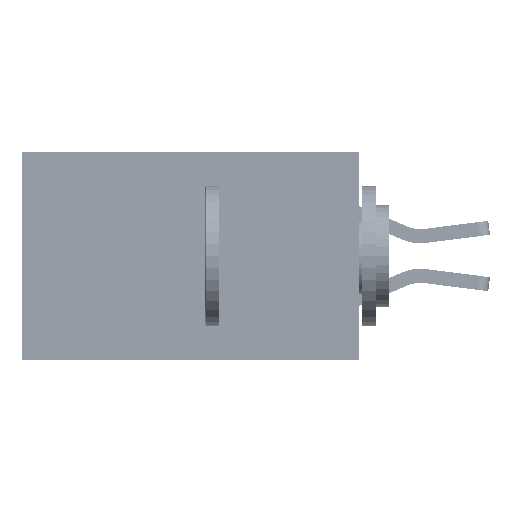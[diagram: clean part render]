
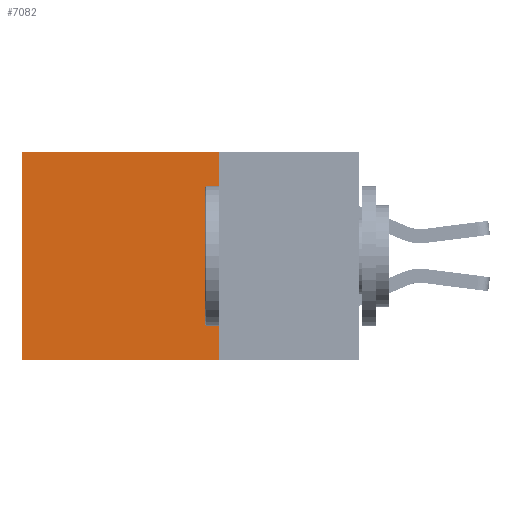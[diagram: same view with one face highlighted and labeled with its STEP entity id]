
A CAD part, left-side view. The second image highlights one B-rep face of the part: STEP entity #7082.
In plain terms, the highlighted planar face has unit normal (-1, 0, 0).
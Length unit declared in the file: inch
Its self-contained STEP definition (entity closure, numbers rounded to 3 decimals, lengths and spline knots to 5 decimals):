
#3027 = EDGE_LOOP ( 'NONE', ( #3146, #21687, #28810, #21002 ) ) ;
#3146 = ORIENTED_EDGE ( 'NONE', *, *, #11453, .T. ) ;
#3350 = EDGE_CURVE ( 'NONE', #18183, #9388, #34153, .T. ) ;
#3653 = VECTOR ( 'NONE', #15631, 39.37008 ) ;
#4981 = DIRECTION ( 'NONE',  ( 0., 0., -1. ) ) ;
#5679 = VERTEX_POINT ( 'NONE', #26186 ) ;
#6028 = CARTESIAN_POINT ( 'NONE',  ( 0.2875, 0.25, -0.37 ) ) ;
#7082 = ADVANCED_FACE ( 'NONE', ( #9370 ), #31191, .F. ) ;
#9370 = FACE_OUTER_BOUND ( 'NONE', #3027, .T. ) ;
#9388 = VERTEX_POINT ( 'NONE', #6028 ) ;
#9707 = CARTESIAN_POINT ( 'NONE',  ( 0.2875, 0.25, 0. ) ) ;
#11453 = EDGE_CURVE ( 'NONE', #5679, #17596, #29459, .T. ) ;
#11769 = CARTESIAN_POINT ( 'NONE',  ( 0.2875, 0.25, 0. ) ) ;
#11948 = DIRECTION ( 'NONE',  ( 0., 0., -1. ) ) ;
#12158 = AXIS2_PLACEMENT_3D ( 'NONE', #34098, #22733, #4981 ) ;
#14828 = DIRECTION ( 'NONE',  ( 0., 0., -1. ) ) ;
#15631 = DIRECTION ( 'NONE',  ( 0., 1., 0. ) ) ;
#17370 = LINE ( 'NONE', #26578, #18271 ) ;
#17596 = VERTEX_POINT ( 'NONE', #35631 ) ;
#18183 = VERTEX_POINT ( 'NONE', #26879 ) ;
#18271 = VECTOR ( 'NONE', #26451, 39.37008 ) ;
#21002 = ORIENTED_EDGE ( 'NONE', *, *, #35787, .T. ) ;
#21687 = ORIENTED_EDGE ( 'NONE', *, *, #34339, .F. ) ;
#22733 = DIRECTION ( 'NONE',  ( 1., 0., 0. ) ) ;
#26186 = CARTESIAN_POINT ( 'NONE',  ( 0.2875, 0.6, 0. ) ) ;
#26224 = LINE ( 'NONE', #9707, #3653 ) ;
#26451 = DIRECTION ( 'NONE',  ( 0., 1., 0. ) ) ;
#26556 = VECTOR ( 'NONE', #14828, 39.37008 ) ;
#26578 = CARTESIAN_POINT ( 'NONE',  ( 0.2875, 0.25, -0.37 ) ) ;
#26879 = CARTESIAN_POINT ( 'NONE',  ( 0.2875, 0.25, 0. ) ) ;
#28810 = ORIENTED_EDGE ( 'NONE', *, *, #3350, .F. ) ;
#29459 = LINE ( 'NONE', #32227, #36158 ) ;
#31191 = PLANE ( 'NONE',  #12158 ) ;
#32227 = CARTESIAN_POINT ( 'NONE',  ( 0.2875, 0.6, 0. ) ) ;
#34098 = CARTESIAN_POINT ( 'NONE',  ( 0.2875, 0.25, 0. ) ) ;
#34153 = LINE ( 'NONE', #11769, #26556 ) ;
#34339 = EDGE_CURVE ( 'NONE', #9388, #17596, #17370, .T. ) ;
#35631 = CARTESIAN_POINT ( 'NONE',  ( 0.2875, 0.6, -0.37 ) ) ;
#35787 = EDGE_CURVE ( 'NONE', #18183, #5679, #26224, .T. ) ;
#36158 = VECTOR ( 'NONE', #11948, 39.37008 ) ;
